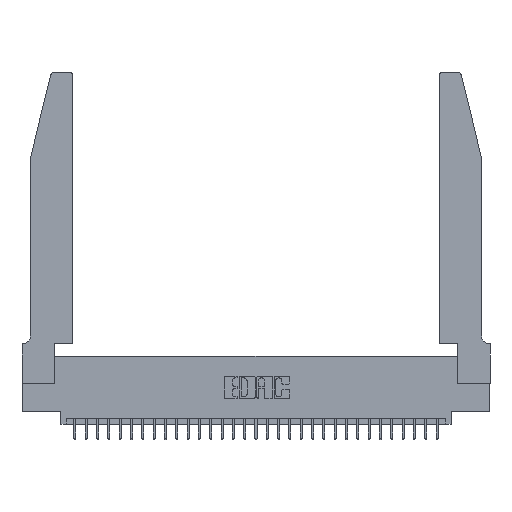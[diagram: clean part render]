
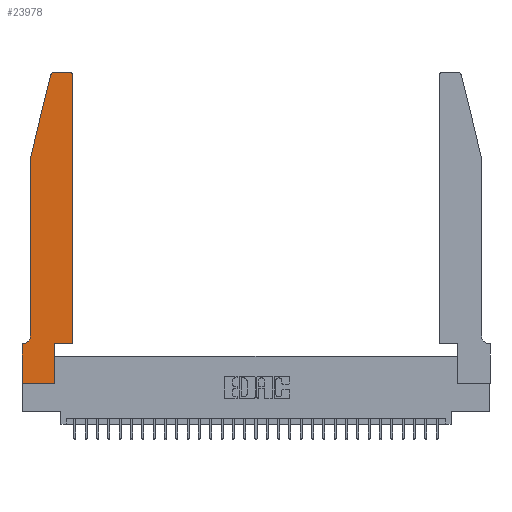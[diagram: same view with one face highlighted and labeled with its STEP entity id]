
A CAD part, top view. The second image highlights one B-rep face of the part: STEP entity #23978.
In plain terms, the highlighted planar face has unit normal (0, 0, 1).
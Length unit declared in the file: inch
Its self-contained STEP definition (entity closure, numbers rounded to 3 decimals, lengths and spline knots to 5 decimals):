
#277 = CIRCLE ( 'NONE', #9093, 0.03 ) ;
#603 = CARTESIAN_POINT ( 'NONE',  ( 0.2865, 0., 0.37 ) ) ;
#987 = DIRECTION ( 'NONE',  ( 0., -1., 0. ) ) ;
#1703 = EDGE_CURVE ( 'NONE', #15276, #24967, #277, .T. ) ;
#1738 = VERTEX_POINT ( 'NONE', #3695 ) ;
#1827 = DIRECTION ( 'NONE',  ( 0., 0., 1. ) ) ;
#2037 = CARTESIAN_POINT ( 'NONE',  ( 0., 0.35, 0.37 ) ) ;
#2188 = CARTESIAN_POINT ( 'NONE',  ( 0.284, 2.72, 0.37 ) ) ;
#2415 = LINE ( 'NONE', #17371, #24072 ) ;
#2425 = CIRCLE ( 'NONE', #15902, 0.07 ) ;
#3154 = DIRECTION ( 'NONE',  ( -0.239, -0.971, 0. ) ) ;
#3176 = DIRECTION ( 'NONE',  ( 1., 0., 0. ) ) ;
#3498 = ORIENTED_EDGE ( 'NONE', *, *, #18545, .T. ) ;
#3543 = VECTOR ( 'NONE', #22503, 39.37008 ) ;
#3695 = CARTESIAN_POINT ( 'NONE',  ( 0.2865, 0.35, 0.37 ) ) ;
#3975 = DIRECTION ( 'NONE',  ( -1., 0., 0. ) ) ;
#4315 = EDGE_CURVE ( 'NONE', #29586, #21317, #32011, .T. ) ;
#4858 = LINE ( 'NONE', #29570, #16396 ) ;
#4907 = DIRECTION ( 'NONE',  ( 1., 0., 0. ) ) ;
#5283 = ORIENTED_EDGE ( 'NONE', *, *, #26646, .T. ) ;
#5440 = CARTESIAN_POINT ( 'NONE',  ( 0.0755, 2., 0.37 ) ) ;
#5966 = DIRECTION ( 'NONE',  ( 0., 1., 0. ) ) ;
#6095 = CARTESIAN_POINT ( 'NONE',  ( 0.0055, 0.42, 0.37 ) ) ;
#6551 = CARTESIAN_POINT ( 'NONE',  ( 0.2605, 2.75, 0.37 ) ) ;
#6657 = VECTOR ( 'NONE', #8466, 39.37008 ) ;
#7070 = DIRECTION ( 'NONE',  ( 0., 0., 1. ) ) ;
#7137 = VERTEX_POINT ( 'NONE', #2037 ) ;
#7249 = CARTESIAN_POINT ( 'NONE',  ( 0.25487, 2.72718, 0.37 ) ) ;
#7402 = ORIENTED_EDGE ( 'NONE', *, *, #21473, .T. ) ;
#7989 = LINE ( 'NONE', #20175, #17300 ) ;
#8466 = DIRECTION ( 'NONE',  ( -1., 0., 0. ) ) ;
#8787 = LINE ( 'NONE', #28627, #6657 ) ;
#9093 = AXIS2_PLACEMENT_3D ( 'NONE', #26458, #14067, #26298 ) ;
#9352 = DIRECTION ( 'NONE',  ( 1., 0., 0. ) ) ;
#10003 = VERTEX_POINT ( 'NONE', #603 ) ;
#10295 = EDGE_CURVE ( 'NONE', #21317, #20866, #25110, .T. ) ;
#10372 = VERTEX_POINT ( 'NONE', #28348 ) ;
#10439 = EDGE_CURVE ( 'NONE', #24967, #29586, #11413, .T. ) ;
#10520 = ORIENTED_EDGE ( 'NONE', *, *, #22862, .T. ) ;
#10840 = VERTEX_POINT ( 'NONE', #10907 ) ;
#10907 = CARTESIAN_POINT ( 'NONE',  ( 0.4505, 0.35, 0.37 ) ) ;
#11413 = LINE ( 'NONE', #6551, #13503 ) ;
#11683 = CARTESIAN_POINT ( 'NONE',  ( 0.0055, 0.35, 0.37 ) ) ;
#12591 = ORIENTED_EDGE ( 'NONE', *, *, #4315, .T. ) ;
#13503 = VECTOR ( 'NONE', #16134, 39.37008 ) ;
#13600 = VERTEX_POINT ( 'NONE', #31345 ) ;
#14067 = DIRECTION ( 'NONE',  ( 0., 0., 1. ) ) ;
#14625 = CARTESIAN_POINT ( 'NONE',  ( 0.4505, 0.35, 0.37 ) ) ;
#14676 = ORIENTED_EDGE ( 'NONE', *, *, #10439, .T. ) ;
#14746 = DIRECTION ( 'NONE',  ( 1., 0., 0. ) ) ;
#15276 = VERTEX_POINT ( 'NONE', #19279 ) ;
#15902 = AXIS2_PLACEMENT_3D ( 'NONE', #6095, #18452, #3975 ) ;
#16134 = DIRECTION ( 'NONE',  ( -1., 0., 0. ) ) ;
#16396 = VECTOR ( 'NONE', #14746, 39.37008 ) ;
#16799 = ORIENTED_EDGE ( 'NONE', *, *, #18757, .T. ) ;
#17300 = VECTOR ( 'NONE', #987, 39.37008 ) ;
#17371 = CARTESIAN_POINT ( 'NONE',  ( 0.2865, 0.35, 0.37 ) ) ;
#17623 = CARTESIAN_POINT ( 'NONE',  ( 0., 0., 0.37 ) ) ;
#18452 = DIRECTION ( 'NONE',  ( 0., 0., -1. ) ) ;
#18545 = EDGE_CURVE ( 'NONE', #10840, #15276, #29457, .T. ) ;
#18757 = EDGE_CURVE ( 'NONE', #20866, #10372, #7989, .T. ) ;
#18964 = VERTEX_POINT ( 'NONE', #11683 ) ;
#18984 = EDGE_CURVE ( 'NONE', #10003, #1738, #2415, .T. ) ;
#19279 = CARTESIAN_POINT ( 'NONE',  ( 0.4505, 2.72, 0.37 ) ) ;
#19303 = ORIENTED_EDGE ( 'NONE', *, *, #18984, .T. ) ;
#19343 = ORIENTED_EDGE ( 'NONE', *, *, #10295, .T. ) ;
#20175 = CARTESIAN_POINT ( 'NONE',  ( 0.0755, 2., 0.37 ) ) ;
#20573 = FACE_OUTER_BOUND ( 'NONE', #27797, .T. ) ;
#20866 = VERTEX_POINT ( 'NONE', #24532 ) ;
#21317 = VERTEX_POINT ( 'NONE', #7249 ) ;
#21473 = EDGE_CURVE ( 'NONE', #13600, #10003, #27891, .T. ) ;
#21972 = DIRECTION ( 'NONE',  ( 0., 1., 0. ) ) ;
#22126 = EDGE_CURVE ( 'NONE', #1738, #10840, #4858, .T. ) ;
#22503 = DIRECTION ( 'NONE',  ( 0., -1., 0. ) ) ;
#22523 = ORIENTED_EDGE ( 'NONE', *, *, #22126, .T. ) ;
#22849 = CARTESIAN_POINT ( 'NONE',  ( 0., 0., 0.37 ) ) ;
#22862 = EDGE_CURVE ( 'NONE', #10372, #18964, #2425, .T. ) ;
#23027 = CARTESIAN_POINT ( 'NONE',  ( 0.4205, 2.75, 0.37 ) ) ;
#23140 = VECTOR ( 'NONE', #3176, 39.37008 ) ;
#23605 = VECTOR ( 'NONE', #21972, 39.37008 ) ;
#23978 = ADVANCED_FACE ( 'NONE', ( #20573 ), #30493, .T. ) ;
#24072 = VECTOR ( 'NONE', #5966, 39.37008 ) ;
#24250 = EDGE_CURVE ( 'NONE', #18964, #7137, #8787, .T. ) ;
#24532 = CARTESIAN_POINT ( 'NONE',  ( 0.0755, 2., 0.37 ) ) ;
#24643 = ORIENTED_EDGE ( 'NONE', *, *, #24250, .T. ) ;
#24967 = VERTEX_POINT ( 'NONE', #23027 ) ;
#25110 = LINE ( 'NONE', #5440, #27030 ) ;
#25513 = ORIENTED_EDGE ( 'NONE', *, *, #1703, .T. ) ;
#26298 = DIRECTION ( 'NONE',  ( 1., 0., 0. ) ) ;
#26384 = CARTESIAN_POINT ( 'NONE',  ( 0., 0.35, 0.37 ) ) ;
#26458 = CARTESIAN_POINT ( 'NONE',  ( 0.4205, 2.72, 0.37 ) ) ;
#26587 = CARTESIAN_POINT ( 'NONE',  ( 0.284, 2.75, 0.37 ) ) ;
#26646 = EDGE_CURVE ( 'NONE', #7137, #13600, #30147, .T. ) ;
#27030 = VECTOR ( 'NONE', #3154, 39.37008 ) ;
#27797 = EDGE_LOOP ( 'NONE', ( #14676, #12591, #19343, #16799, #10520, #24643, #5283, #7402, #19303, #22523, #3498, #25513 ) ) ;
#27891 = LINE ( 'NONE', #22849, #23140 ) ;
#28348 = CARTESIAN_POINT ( 'NONE',  ( 0.0755, 0.42, 0.37 ) ) ;
#28627 = CARTESIAN_POINT ( 'NONE',  ( 0.0755, 0.35, 0.37 ) ) ;
#29457 = LINE ( 'NONE', #14625, #23605 ) ;
#29462 = AXIS2_PLACEMENT_3D ( 'NONE', #2188, #7070, #9352 ) ;
#29471 = AXIS2_PLACEMENT_3D ( 'NONE', #26384, #1827, #4907 ) ;
#29570 = CARTESIAN_POINT ( 'NONE',  ( 0.4505, 0.35, 0.37 ) ) ;
#29586 = VERTEX_POINT ( 'NONE', #26587 ) ;
#30147 = LINE ( 'NONE', #17623, #3543 ) ;
#30493 = PLANE ( 'NONE',  #29471 ) ;
#31345 = CARTESIAN_POINT ( 'NONE',  ( 0., 0., 0.37 ) ) ;
#32011 = CIRCLE ( 'NONE', #29462, 0.03 ) ;
